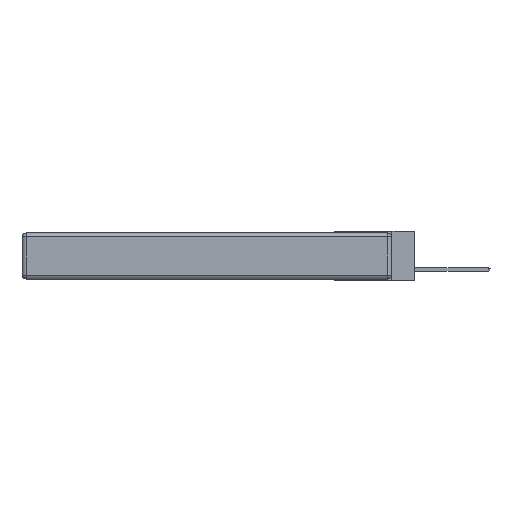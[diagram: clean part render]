
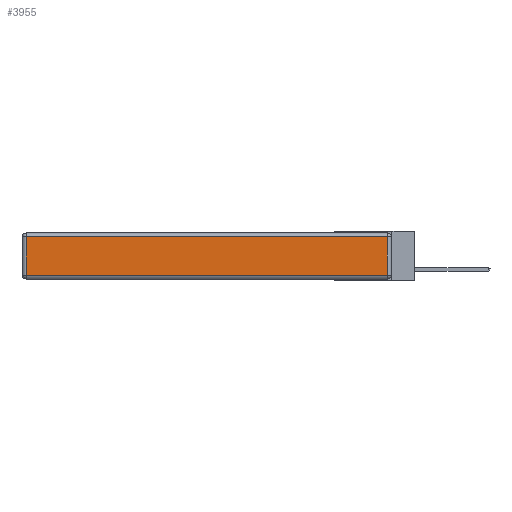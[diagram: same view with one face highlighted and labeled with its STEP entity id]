
A CAD part, left-side view. The second image highlights one B-rep face of the part: STEP entity #3955.
In plain terms, the highlighted planar face has unit normal (-1, 0, 0).
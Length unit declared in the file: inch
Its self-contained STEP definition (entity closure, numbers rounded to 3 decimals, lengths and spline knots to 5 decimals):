
#215 = EDGE_LOOP ( 'NONE', ( #20415, #5576, #18809, #17727 ) ) ;
#1035 = VECTOR ( 'NONE', #14390, 39.37008 ) ;
#1084 = DIRECTION ( 'NONE',  ( 0., -1., 0. ) ) ;
#2035 = VERTEX_POINT ( 'NONE', #16144 ) ;
#3755 = PLANE ( 'NONE',  #12956 ) ;
#3955 = ADVANCED_FACE ( 'NONE', ( #17339 ), #3755, .T. ) ;
#4742 = CARTESIAN_POINT ( 'NONE',  ( 0., 0.03, -0.03 ) ) ;
#5066 = VERTEX_POINT ( 'NONE', #13570 ) ;
#5258 = CARTESIAN_POINT ( 'NONE',  ( 0., 0., -0.343 ) ) ;
#5576 = ORIENTED_EDGE ( 'NONE', *, *, #17061, .T. ) ;
#5591 = EDGE_CURVE ( 'NONE', #14351, #5066, #8592, .T. ) ;
#5932 = CARTESIAN_POINT ( 'NONE',  ( 0., 2.75, -0.03 ) ) ;
#6177 = CARTESIAN_POINT ( 'NONE',  ( 0., 0.03, -0.343 ) ) ;
#7513 = CARTESIAN_POINT ( 'NONE',  ( 0., 0., -0.313 ) ) ;
#7637 = EDGE_CURVE ( 'NONE', #5066, #2035, #9423, .T. ) ;
#8273 = DIRECTION ( 'NONE',  ( 0., 0., 1. ) ) ;
#8489 = VERTEX_POINT ( 'NONE', #4742 ) ;
#8592 = LINE ( 'NONE', #12225, #9318 ) ;
#8779 = EDGE_CURVE ( 'NONE', #8489, #14351, #15388, .T. ) ;
#9318 = VECTOR ( 'NONE', #12161, 39.37008 ) ;
#9423 = LINE ( 'NONE', #7513, #10708 ) ;
#10708 = VECTOR ( 'NONE', #1084, 39.37008 ) ;
#11163 = VECTOR ( 'NONE', #18661, 39.37008 ) ;
#12161 = DIRECTION ( 'NONE',  ( 0., 0., -1. ) ) ;
#12225 = CARTESIAN_POINT ( 'NONE',  ( 0., 2.72, -0.343 ) ) ;
#12956 = AXIS2_PLACEMENT_3D ( 'NONE', #5258, #13157, #8273 ) ;
#13157 = DIRECTION ( 'NONE',  ( -1., 0., 0. ) ) ;
#13570 = CARTESIAN_POINT ( 'NONE',  ( 0., 2.72, -0.313 ) ) ;
#14351 = VERTEX_POINT ( 'NONE', #17870 ) ;
#14390 = DIRECTION ( 'NONE',  ( 0., 0., 1. ) ) ;
#15388 = LINE ( 'NONE', #5932, #11163 ) ;
#16144 = CARTESIAN_POINT ( 'NONE',  ( 0., 0.03, -0.313 ) ) ;
#17061 = EDGE_CURVE ( 'NONE', #2035, #8489, #17446, .T. ) ;
#17339 = FACE_OUTER_BOUND ( 'NONE', #215, .T. ) ;
#17446 = LINE ( 'NONE', #6177, #1035 ) ;
#17727 = ORIENTED_EDGE ( 'NONE', *, *, #5591, .T. ) ;
#17870 = CARTESIAN_POINT ( 'NONE',  ( 0., 2.72, -0.03 ) ) ;
#18661 = DIRECTION ( 'NONE',  ( 0., 1., 0. ) ) ;
#18809 = ORIENTED_EDGE ( 'NONE', *, *, #8779, .T. ) ;
#20415 = ORIENTED_EDGE ( 'NONE', *, *, #7637, .T. ) ;
